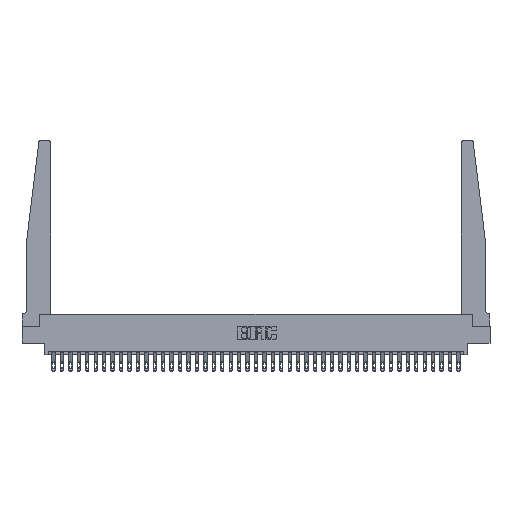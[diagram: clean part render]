
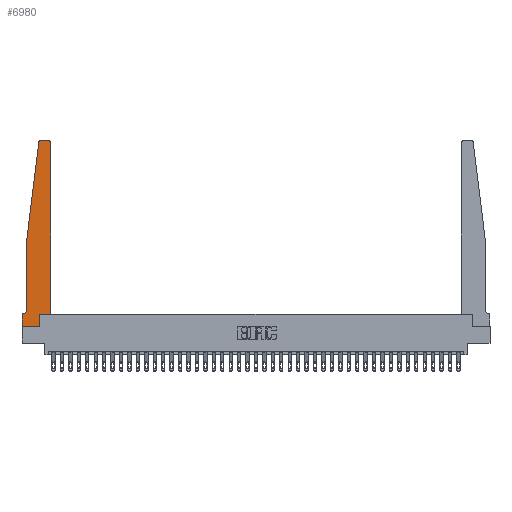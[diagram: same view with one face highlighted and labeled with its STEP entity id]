
A CAD part, top view. The second image highlights one B-rep face of the part: STEP entity #6980.
In plain terms, the highlighted planar face has unit normal (0, 0, 1).
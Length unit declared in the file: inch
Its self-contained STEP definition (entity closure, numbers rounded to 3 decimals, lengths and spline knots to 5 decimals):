
#1858 = EDGE_CURVE ( 'NONE', #9593, #10128, #7578, .T. ) ;
#2065 = CARTESIAN_POINT ( 'NONE',  ( 0.065, 0.1875, 0.37 ) ) ;
#2072 = VERTEX_POINT ( 'NONE', #11509 ) ;
#2541 = EDGE_CURVE ( 'NONE', #2072, #26841, #8284, .T. ) ;
#2763 = CARTESIAN_POINT ( 'NONE',  ( 0.395, 2.72, 0.37 ) ) ;
#2968 = ORIENTED_EDGE ( 'NONE', *, *, #5409, .T. ) ;
#3007 = VERTEX_POINT ( 'NONE', #31529 ) ;
#3014 = VERTEX_POINT ( 'NONE', #17404 ) ;
#3322 = ORIENTED_EDGE ( 'NONE', *, *, #35052, .T. ) ;
#3362 = VERTEX_POINT ( 'NONE', #31479 ) ;
#3448 = DIRECTION ( 'NONE',  ( -0.122, -0.992, 0. ) ) ;
#3690 = ORIENTED_EDGE ( 'NONE', *, *, #5996, .T. ) ;
#4237 = DIRECTION ( 'NONE',  ( -1., 0., 0. ) ) ;
#4310 = ORIENTED_EDGE ( 'NONE', *, *, #2541, .T. ) ;
#4807 = CARTESIAN_POINT ( 'NONE',  ( 0.065, 1.25, 0.37 ) ) ;
#5265 = CARTESIAN_POINT ( 'NONE',  ( 0.2605, 0.18, 0.37 ) ) ;
#5409 = EDGE_CURVE ( 'NONE', #26841, #29601, #11121, .T. ) ;
#5901 = DIRECTION ( 'NONE',  ( 1., 0., 0. ) ) ;
#5996 = EDGE_CURVE ( 'NONE', #10128, #3007, #14587, .T. ) ;
#6249 = ORIENTED_EDGE ( 'NONE', *, *, #21801, .T. ) ;
#6258 = AXIS2_PLACEMENT_3D ( 'NONE', #14045, #25413, #16311 ) ;
#6505 = ORIENTED_EDGE ( 'NONE', *, *, #1858, .T. ) ;
#6980 = ADVANCED_FACE ( 'NONE', ( #11685 ), #34554, .T. ) ;
#7528 = VECTOR ( 'NONE', #31014, 39.37008 ) ;
#7578 = LINE ( 'NONE', #4807, #32113 ) ;
#7775 = DIRECTION ( 'NONE',  ( 0., 0., 1. ) ) ;
#7920 = EDGE_CURVE ( 'NONE', #3362, #28592, #36618, .T. ) ;
#8284 = LINE ( 'NONE', #25416, #7528 ) ;
#8690 = DIRECTION ( 'NONE',  ( 0., 0., 1. ) ) ;
#8943 = VECTOR ( 'NONE', #4237, 39.37008 ) ;
#9214 = CARTESIAN_POINT ( 'NONE',  ( 0., 0., 0.37 ) ) ;
#9593 = VERTEX_POINT ( 'NONE', #34718 ) ;
#10128 = VERTEX_POINT ( 'NONE', #12726 ) ;
#10686 = CARTESIAN_POINT ( 'NONE',  ( 0.2605, 0., 0.37 ) ) ;
#10710 = EDGE_CURVE ( 'NONE', #3007, #3362, #24771, .T. ) ;
#11121 = LINE ( 'NONE', #30508, #22854 ) ;
#11446 = VERTEX_POINT ( 'NONE', #10686 ) ;
#11509 = CARTESIAN_POINT ( 'NONE',  ( 0.2605, 0.18, 0.37 ) ) ;
#11535 = ORIENTED_EDGE ( 'NONE', *, *, #16378, .T. ) ;
#11685 = FACE_OUTER_BOUND ( 'NONE', #13807, .T. ) ;
#12543 = VECTOR ( 'NONE', #28649, 39.37008 ) ;
#12726 = CARTESIAN_POINT ( 'NONE',  ( 0.065, 0.2375, 0.37 ) ) ;
#13413 = DIRECTION ( 'NONE',  ( -1., 0., 0. ) ) ;
#13807 = EDGE_LOOP ( 'NONE', ( #6249, #3322, #11535, #6505, #3690, #35914, #16362, #22465, #33558, #4310, #2968, #14941 ) ) ;
#14045 = CARTESIAN_POINT ( 'NONE',  ( 0.015, 0.2375, 0.37 ) ) ;
#14587 = CIRCLE ( 'NONE', #6258, 0.05 ) ;
#14941 = ORIENTED_EDGE ( 'NONE', *, *, #15784, .T. ) ;
#15063 = DIRECTION ( 'NONE',  ( 1., 0., 0. ) ) ;
#15784 = EDGE_CURVE ( 'NONE', #29601, #34941, #23010, .T. ) ;
#16311 = DIRECTION ( 'NONE',  ( -1., 0., 0. ) ) ;
#16362 = ORIENTED_EDGE ( 'NONE', *, *, #7920, .T. ) ;
#16378 = EDGE_CURVE ( 'NONE', #19633, #9593, #20229, .T. ) ;
#16939 = CARTESIAN_POINT ( 'NONE',  ( 0., 0., 0.37 ) ) ;
#17404 = CARTESIAN_POINT ( 'NONE',  ( 0.27653, 2.75, 0.37 ) ) ;
#18411 = LINE ( 'NONE', #20839, #8943 ) ;
#18434 = DIRECTION ( 'NONE',  ( 1., 0., 0. ) ) ;
#19183 = DIRECTION ( 'NONE',  ( 1., 0., 0. ) ) ;
#19509 = AXIS2_PLACEMENT_3D ( 'NONE', #27137, #32540, #18434 ) ;
#19633 = VERTEX_POINT ( 'NONE', #24074 ) ;
#19721 = DIRECTION ( 'NONE',  ( 0., 1., 0. ) ) ;
#20229 = LINE ( 'NONE', #31559, #28364 ) ;
#20488 = VECTOR ( 'NONE', #15063, 39.37008 ) ;
#20517 = CARTESIAN_POINT ( 'NONE',  ( 0.425, 2.72, 0.37 ) ) ;
#20619 = AXIS2_PLACEMENT_3D ( 'NONE', #2763, #7775, #19183 ) ;
#20658 = LINE ( 'NONE', #31990, #20488 ) ;
#20839 = CARTESIAN_POINT ( 'NONE',  ( 0.25, 2.75, 0.37 ) ) ;
#20948 = VECTOR ( 'NONE', #33720, 39.37008 ) ;
#21801 = EDGE_CURVE ( 'NONE', #34941, #3014, #18411, .T. ) ;
#22014 = CARTESIAN_POINT ( 'NONE',  ( 0.425, 0.18, 0.37 ) ) ;
#22465 = ORIENTED_EDGE ( 'NONE', *, *, #30329, .T. ) ;
#22854 = VECTOR ( 'NONE', #19721, 39.37008 ) ;
#23010 = CIRCLE ( 'NONE', #20619, 0.03 ) ;
#23246 = VECTOR ( 'NONE', #13413, 39.37008 ) ;
#23716 = EDGE_CURVE ( 'NONE', #11446, #2072, #30963, .T. ) ;
#24074 = CARTESIAN_POINT ( 'NONE',  ( 0.24675, 2.72367, 0.37 ) ) ;
#24771 = LINE ( 'NONE', #2065, #23246 ) ;
#25413 = DIRECTION ( 'NONE',  ( 0., 0., -1. ) ) ;
#25416 = CARTESIAN_POINT ( 'NONE',  ( 0.425, 0.18, 0.37 ) ) ;
#26841 = VERTEX_POINT ( 'NONE', #22014 ) ;
#27137 = CARTESIAN_POINT ( 'NONE',  ( 0.27653, 2.72, 0.37 ) ) ;
#27891 = DIRECTION ( 'NONE',  ( 0., -1., 0. ) ) ;
#28364 = VECTOR ( 'NONE', #3448, 39.37008 ) ;
#28592 = VERTEX_POINT ( 'NONE', #9214 ) ;
#28649 = DIRECTION ( 'NONE',  ( 0., -1., 0. ) ) ;
#29399 = CARTESIAN_POINT ( 'NONE',  ( 0.395, 2.75, 0.37 ) ) ;
#29601 = VERTEX_POINT ( 'NONE', #20517 ) ;
#30329 = EDGE_CURVE ( 'NONE', #28592, #11446, #20658, .T. ) ;
#30508 = CARTESIAN_POINT ( 'NONE',  ( 0.425, 0.18, 0.37 ) ) ;
#30788 = CIRCLE ( 'NONE', #19509, 0.03 ) ;
#30963 = LINE ( 'NONE', #5265, #20948 ) ;
#31014 = DIRECTION ( 'NONE',  ( 1., 0., 0. ) ) ;
#31479 = CARTESIAN_POINT ( 'NONE',  ( 0., 0.1875, 0.37 ) ) ;
#31529 = CARTESIAN_POINT ( 'NONE',  ( 0.015, 0.1875, 0.37 ) ) ;
#31559 = CARTESIAN_POINT ( 'NONE',  ( 0.065, 1.25, 0.37 ) ) ;
#31990 = CARTESIAN_POINT ( 'NONE',  ( 0., 0., 0.37 ) ) ;
#32113 = VECTOR ( 'NONE', #27891, 39.37008 ) ;
#32540 = DIRECTION ( 'NONE',  ( 0., 0., 1. ) ) ;
#33114 = AXIS2_PLACEMENT_3D ( 'NONE', #34178, #8690, #5901 ) ;
#33558 = ORIENTED_EDGE ( 'NONE', *, *, #23716, .T. ) ;
#33720 = DIRECTION ( 'NONE',  ( 0., 1., 0. ) ) ;
#34178 = CARTESIAN_POINT ( 'NONE',  ( 0., 0.1875, 0.37 ) ) ;
#34554 = PLANE ( 'NONE',  #33114 ) ;
#34718 = CARTESIAN_POINT ( 'NONE',  ( 0.065, 1.25, 0.37 ) ) ;
#34941 = VERTEX_POINT ( 'NONE', #29399 ) ;
#35052 = EDGE_CURVE ( 'NONE', #3014, #19633, #30788, .T. ) ;
#35914 = ORIENTED_EDGE ( 'NONE', *, *, #10710, .T. ) ;
#36618 = LINE ( 'NONE', #16939, #12543 ) ;
